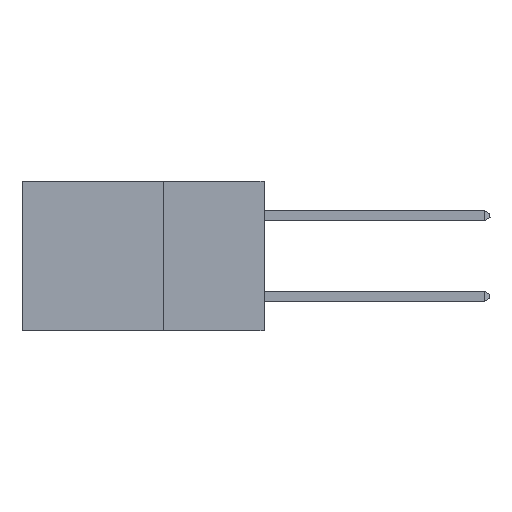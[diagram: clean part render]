
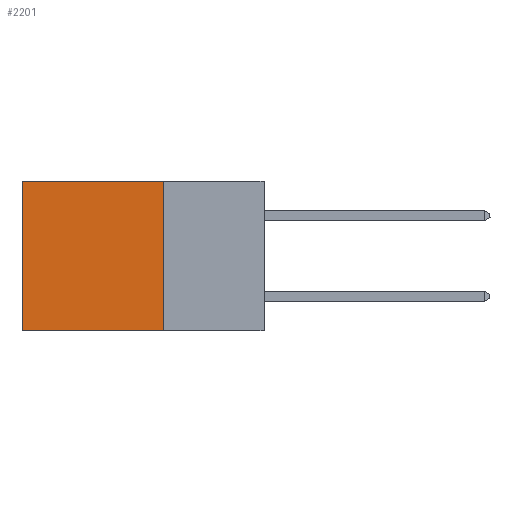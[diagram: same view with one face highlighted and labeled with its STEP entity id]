
A CAD part, left-side view. The second image highlights one B-rep face of the part: STEP entity #2201.
In plain terms, the highlighted planar face has unit normal (-1, 0, 0).
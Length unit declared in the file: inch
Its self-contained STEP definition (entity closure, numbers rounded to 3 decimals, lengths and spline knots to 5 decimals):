
#373 = LINE ( 'NONE', #17611, #3210 ) ;
#2201 = ADVANCED_FACE ( 'NONE', ( #2789 ), #7430, .F. ) ;
#2301 = LINE ( 'NONE', #9599, #16156 ) ;
#2751 = VERTEX_POINT ( 'NONE', #9888 ) ;
#2789 = FACE_OUTER_BOUND ( 'NONE', #8481, .T. ) ;
#3210 = VECTOR ( 'NONE', #21310, 39.37008 ) ;
#3488 = CARTESIAN_POINT ( 'NONE',  ( 0.298, 0.6, 0. ) ) ;
#3965 = ORIENTED_EDGE ( 'NONE', *, *, #7280, .T. ) ;
#4815 = AXIS2_PLACEMENT_3D ( 'NONE', #18544, #12938, #13150 ) ;
#6731 = CARTESIAN_POINT ( 'NONE',  ( 0.298, 0.25, -0.37 ) ) ;
#7180 = ORIENTED_EDGE ( 'NONE', *, *, #21672, .F. ) ;
#7280 = EDGE_CURVE ( 'NONE', #2751, #19299, #373, .T. ) ;
#7430 = PLANE ( 'NONE',  #4815 ) ;
#7776 = VECTOR ( 'NONE', #10583, 39.37008 ) ;
#8481 = EDGE_LOOP ( 'NONE', ( #22606, #7180, #14098, #3965 ) ) ;
#9281 = VERTEX_POINT ( 'NONE', #15985 ) ;
#9599 = CARTESIAN_POINT ( 'NONE',  ( 0.298, 0.25, 0. ) ) ;
#9888 = CARTESIAN_POINT ( 'NONE',  ( 0.298, 0.25, 0. ) ) ;
#10583 = DIRECTION ( 'NONE',  ( 0., 0., -1. ) ) ;
#11175 = LINE ( 'NONE', #3488, #7776 ) ;
#12067 = DIRECTION ( 'NONE',  ( 0., 1., 0. ) ) ;
#12233 = EDGE_CURVE ( 'NONE', #2751, #13599, #2301, .T. ) ;
#12938 = DIRECTION ( 'NONE',  ( 1., 0., 0. ) ) ;
#13150 = DIRECTION ( 'NONE',  ( 0., 0., -1. ) ) ;
#13599 = VERTEX_POINT ( 'NONE', #19450 ) ;
#14098 = ORIENTED_EDGE ( 'NONE', *, *, #12233, .F. ) ;
#15985 = CARTESIAN_POINT ( 'NONE',  ( 0.298, 0.6, -0.37 ) ) ;
#16042 = EDGE_CURVE ( 'NONE', #19299, #9281, #11175, .T. ) ;
#16156 = VECTOR ( 'NONE', #16534, 39.37008 ) ;
#16534 = DIRECTION ( 'NONE',  ( 0., 0., -1. ) ) ;
#17611 = CARTESIAN_POINT ( 'NONE',  ( 0.298, 0.25, 0. ) ) ;
#18544 = CARTESIAN_POINT ( 'NONE',  ( 0.298, 0.25, 0. ) ) ;
#19299 = VERTEX_POINT ( 'NONE', #21285 ) ;
#19450 = CARTESIAN_POINT ( 'NONE',  ( 0.298, 0.25, -0.37 ) ) ;
#20220 = VECTOR ( 'NONE', #12067, 39.37008 ) ;
#21285 = CARTESIAN_POINT ( 'NONE',  ( 0.298, 0.6, 0. ) ) ;
#21310 = DIRECTION ( 'NONE',  ( 0., 1., 0. ) ) ;
#21672 = EDGE_CURVE ( 'NONE', #13599, #9281, #22476, .T. ) ;
#22476 = LINE ( 'NONE', #6731, #20220 ) ;
#22606 = ORIENTED_EDGE ( 'NONE', *, *, #16042, .T. ) ;
